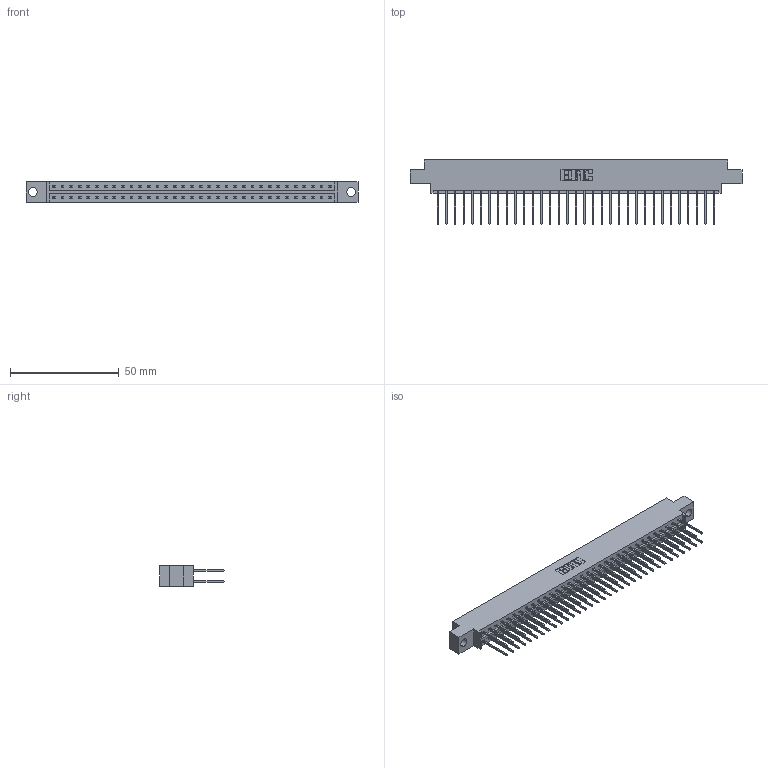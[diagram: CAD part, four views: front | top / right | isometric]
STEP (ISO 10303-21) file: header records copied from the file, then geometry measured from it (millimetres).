
FILE_DESCRIPTION (( 'STEP AP203' ), '1' );
FILE_NAME ('833-066-540-804.STEP', '2020-06-05T08:54:13', ( '' ), ( '' ), 'SwSTEP 2.0', 'SolidWorks 2020', '' );
FILE_SCHEMA (( 'CONFIG_CONTROL_DESIGN' ));
Length unit declared in the file: inch
Products named in the file (3): 833-066-540-804; 345-292-001_345-293-140; 833 Part_Offset - .156 Dia - TH
Assembly tree (67 placements, depth 2):
  833-066-540-804
    833 Part_Offset - .156 Dia - TH
    345-292-001_345-293-140  x66
Bounding box: 152.3 x 29.47 x 9.4 mm (x, y, z)
Volume: 15399.2 mm3; surface area: 19357.5 mm2
Topology: 67 solids, 67 shells, 3550 faces, 10553 edges, 6946 vertices
Faces by surface type: plane 2450, cylinder 1100
Entity records: 22547 total; most frequent: CARTESIAN_POINT 3750, ORIENTED_EDGE 3686, DIRECTION 3219, EDGE_CURVE 1843, VECTOR 1715, LINE 1715, VERTEX_POINT 1226, AXIS2_PLACEMENT_3D 752
